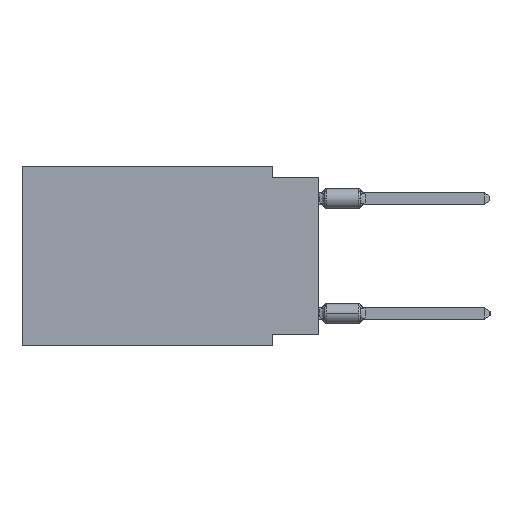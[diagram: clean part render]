
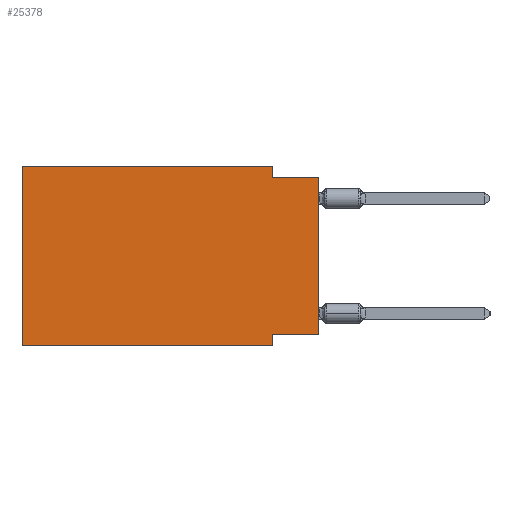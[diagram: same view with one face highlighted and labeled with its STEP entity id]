
A CAD part, left-side view. The second image highlights one B-rep face of the part: STEP entity #25378.
In plain terms, the highlighted planar face has unit normal (-1, 0, 0).
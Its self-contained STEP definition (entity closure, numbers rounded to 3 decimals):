
#109 = ORIENTED_EDGE ( 'NONE', *, *, #29508, .F. ) ;
#263 = EDGE_CURVE ( 'NONE', #17114, #24908, #22109, .T. ) ;
#779 = CARTESIAN_POINT ( 'NONE',  ( 0., 16.383, 0. ) ) ;
#894 = ORIENTED_EDGE ( 'NONE', *, *, #37162, .F. ) ;
#1440 = CARTESIAN_POINT ( 'NONE',  ( 0., 16.383, 0. ) ) ;
#1765 = VECTOR ( 'NONE', #34726, 1000. ) ;
#2543 = DIRECTION ( 'NONE',  ( 0., -1., 0. ) ) ;
#2549 = DIRECTION ( 'NONE',  ( 0., 0., 1. ) ) ;
#2832 = EDGE_CURVE ( 'NONE', #17921, #32074, #18134, .T. ) ;
#3197 = VERTEX_POINT ( 'NONE', #3477 ) ;
#3477 = CARTESIAN_POINT ( 'NONE',  ( 0., 2.54, -9.271 ) ) ;
#3600 = VECTOR ( 'NONE', #23318, 1000. ) ;
#3896 = ORIENTED_EDGE ( 'NONE', *, *, #9900, .F. ) ;
#4600 = DIRECTION ( 'NONE',  ( 0., 0., -1. ) ) ;
#4873 = EDGE_CURVE ( 'NONE', #3197, #22723, #13317, .T. ) ;
#5903 = EDGE_CURVE ( 'NONE', #16817, #24908, #32953, .T. ) ;
#7651 = CARTESIAN_POINT ( 'NONE',  ( 0., 0., -0.635 ) ) ;
#9900 = EDGE_CURVE ( 'NONE', #31887, #17921, #34491, .T. ) ;
#10522 = LINE ( 'NONE', #23125, #3600 ) ;
#10592 = EDGE_LOOP ( 'NONE', ( #19967, #15999, #894, #28697, #3896, #31518, #23464, #109 ) ) ;
#11604 = CARTESIAN_POINT ( 'NONE',  ( 0., 0., -9.271 ) ) ;
#12225 = CARTESIAN_POINT ( 'NONE',  ( 0., 2.54, -9.906 ) ) ;
#13317 = LINE ( 'NONE', #22511, #1765 ) ;
#13454 = DIRECTION ( 'NONE',  ( 0., 0., 1. ) ) ;
#14053 = LINE ( 'NONE', #14450, #35896 ) ;
#14450 = CARTESIAN_POINT ( 'NONE',  ( 0., 2.54, 0. ) ) ;
#15705 = VECTOR ( 'NONE', #13454, 1000. ) ;
#15999 = ORIENTED_EDGE ( 'NONE', *, *, #263, .F. ) ;
#16535 = VECTOR ( 'NONE', #2549, 1000. ) ;
#16670 = CARTESIAN_POINT ( 'NONE',  ( 0., 2.54, 0. ) ) ;
#16817 = VERTEX_POINT ( 'NONE', #18753 ) ;
#17026 = VECTOR ( 'NONE', #27013, 1000. ) ;
#17051 = DIRECTION ( 'NONE',  ( 0., 0., -1. ) ) ;
#17114 = VERTEX_POINT ( 'NONE', #33740 ) ;
#17921 = VERTEX_POINT ( 'NONE', #779 ) ;
#18134 = LINE ( 'NONE', #29965, #24928 ) ;
#18753 = CARTESIAN_POINT ( 'NONE',  ( 0., 0., -9.271 ) ) ;
#19967 = ORIENTED_EDGE ( 'NONE', *, *, #5903, .T. ) ;
#19983 = PLANE ( 'NONE',  #30630 ) ;
#20355 = VECTOR ( 'NONE', #31354, 1000. ) ;
#22109 = LINE ( 'NONE', #22320, #20355 ) ;
#22320 = CARTESIAN_POINT ( 'NONE',  ( 0., 0., -0.635 ) ) ;
#22511 = CARTESIAN_POINT ( 'NONE',  ( 0., 2.54, -9.906 ) ) ;
#22723 = VERTEX_POINT ( 'NONE', #12225 ) ;
#23125 = CARTESIAN_POINT ( 'NONE',  ( 0., 16.383, -9.906 ) ) ;
#23318 = DIRECTION ( 'NONE',  ( 0., -1., 0. ) ) ;
#23464 = ORIENTED_EDGE ( 'NONE', *, *, #4873, .F. ) ;
#24143 = CARTESIAN_POINT ( 'NONE',  ( 0., 0., 0. ) ) ;
#24908 = VERTEX_POINT ( 'NONE', #7651 ) ;
#24928 = VECTOR ( 'NONE', #2543, 1000. ) ;
#25378 = ADVANCED_FACE ( 'NONE', ( #28631 ), #19983, .F. ) ;
#25607 = DIRECTION ( 'NONE',  ( 1., 0., 0. ) ) ;
#27013 = DIRECTION ( 'NONE',  ( 0., 1., 0. ) ) ;
#28631 = FACE_OUTER_BOUND ( 'NONE', #10592, .T. ) ;
#28697 = ORIENTED_EDGE ( 'NONE', *, *, #2832, .F. ) ;
#29508 = EDGE_CURVE ( 'NONE', #16817, #3197, #36023, .T. ) ;
#29965 = CARTESIAN_POINT ( 'NONE',  ( 0., 16.383, 0. ) ) ;
#30630 = AXIS2_PLACEMENT_3D ( 'NONE', #35226, #25607, #4600 ) ;
#31354 = DIRECTION ( 'NONE',  ( 0., -1., 0. ) ) ;
#31518 = ORIENTED_EDGE ( 'NONE', *, *, #34668, .T. ) ;
#31887 = VERTEX_POINT ( 'NONE', #32529 ) ;
#32074 = VERTEX_POINT ( 'NONE', #16670 ) ;
#32529 = CARTESIAN_POINT ( 'NONE',  ( 0., 16.383, -9.906 ) ) ;
#32953 = LINE ( 'NONE', #24143, #16535 ) ;
#33740 = CARTESIAN_POINT ( 'NONE',  ( 0., 2.54, -0.635 ) ) ;
#34491 = LINE ( 'NONE', #1440, #15705 ) ;
#34668 = EDGE_CURVE ( 'NONE', #31887, #22723, #10522, .T. ) ;
#34726 = DIRECTION ( 'NONE',  ( 0., 0., -1. ) ) ;
#35226 = CARTESIAN_POINT ( 'NONE',  ( 0., 16.383, 0. ) ) ;
#35896 = VECTOR ( 'NONE', #17051, 1000. ) ;
#36023 = LINE ( 'NONE', #11604, #17026 ) ;
#37162 = EDGE_CURVE ( 'NONE', #32074, #17114, #14053, .T. ) ;
